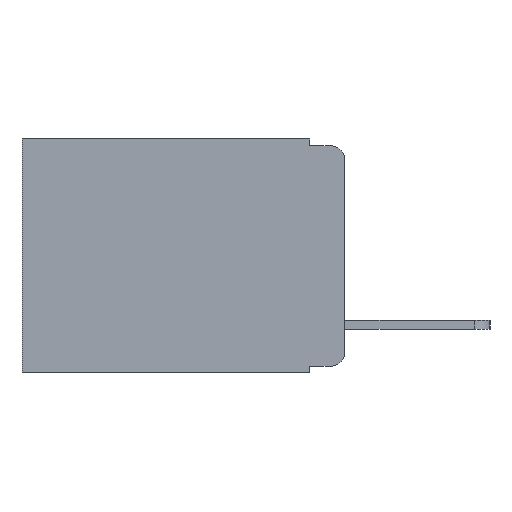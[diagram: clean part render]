
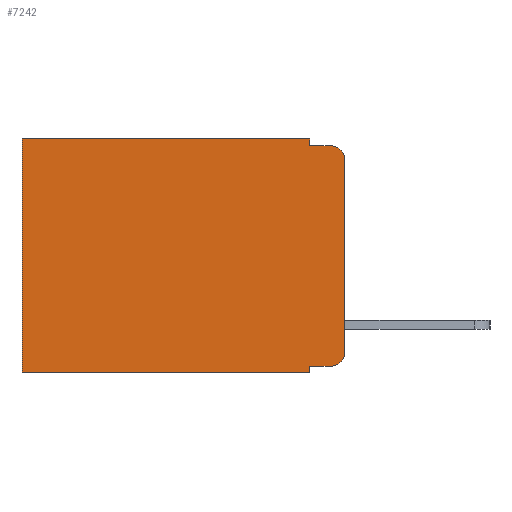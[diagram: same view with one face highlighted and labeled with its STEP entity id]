
A CAD part, left-side view. The second image highlights one B-rep face of the part: STEP entity #7242.
In plain terms, the highlighted planar face has unit normal (-1, 0, 0).
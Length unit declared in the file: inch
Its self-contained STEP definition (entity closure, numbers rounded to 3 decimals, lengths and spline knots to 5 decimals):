
#86 = EDGE_CURVE ( 'NONE', #5661, #2500, #11381, .T. ) ;
#133 = EDGE_LOOP ( 'NONE', ( #2097, #4740, #5464, #5956, #7734, #8742, #486, #1906, #2300, #2674 ) ) ;
#258 = VECTOR ( 'NONE', #10745, 39.37008 ) ;
#445 = VERTEX_POINT ( 'NONE', #5318 ) ;
#486 = ORIENTED_EDGE ( 'NONE', *, *, #9633, .F. ) ;
#683 = LINE ( 'NONE', #10612, #258 ) ;
#869 = VECTOR ( 'NONE', #9114, 39.37008 ) ;
#886 = LINE ( 'NONE', #9125, #869 ) ;
#1081 = DIRECTION ( 'NONE',  ( 0., 0., -1. ) ) ;
#1090 = EDGE_CURVE ( 'NONE', #4045, #10059, #2312, .T. ) ;
#1154 = DIRECTION ( 'NONE',  ( -1., 0., 0. ) ) ;
#1195 = CARTESIAN_POINT ( 'NONE',  ( 0.298, 0.02, -0.03 ) ) ;
#1906 = ORIENTED_EDGE ( 'NONE', *, *, #3934, .F. ) ;
#2074 = VECTOR ( 'NONE', #3559, 39.37008 ) ;
#2097 = ORIENTED_EDGE ( 'NONE', *, *, #8416, .F. ) ;
#2136 = LINE ( 'NONE', #9991, #2074 ) ;
#2219 = AXIS2_PLACEMENT_3D ( 'NONE', #10887, #10707, #10687 ) ;
#2300 = ORIENTED_EDGE ( 'NONE', *, *, #5698, .T. ) ;
#2312 = CIRCLE ( 'NONE', #11860, 0.02 ) ;
#2500 = VERTEX_POINT ( 'NONE', #11569 ) ;
#2591 = EDGE_CURVE ( 'NONE', #4491, #2834, #9206, .T. ) ;
#2674 = ORIENTED_EDGE ( 'NONE', *, *, #1090, .T. ) ;
#2834 = VERTEX_POINT ( 'NONE', #4351 ) ;
#3559 = DIRECTION ( 'NONE',  ( 0., -1., 0. ) ) ;
#3733 = VERTEX_POINT ( 'NONE', #9116 ) ;
#3934 = EDGE_CURVE ( 'NONE', #445, #3733, #886, .T. ) ;
#3970 = CIRCLE ( 'NONE', #11551, 0.02 ) ;
#4045 = VERTEX_POINT ( 'NONE', #9302 ) ;
#4310 = CARTESIAN_POINT ( 'NONE',  ( 0.298, 0., -0.03 ) ) ;
#4351 = CARTESIAN_POINT ( 'NONE',  ( 0.298, 0.473, -0.343 ) ) ;
#4491 = VERTEX_POINT ( 'NONE', #7761 ) ;
#4510 = VERTEX_POINT ( 'NONE', #4310 ) ;
#4536 = EDGE_CURVE ( 'NONE', #7663, #5661, #7298, .T. ) ;
#4740 = ORIENTED_EDGE ( 'NONE', *, *, #9412, .T. ) ;
#4884 = DIRECTION ( 'NONE',  ( 0., -1., 0. ) ) ;
#5318 = CARTESIAN_POINT ( 'NONE',  ( 0.298, 0.051, -0.333 ) ) ;
#5464 = ORIENTED_EDGE ( 'NONE', *, *, #86, .F. ) ;
#5661 = VERTEX_POINT ( 'NONE', #8100 ) ;
#5698 = EDGE_CURVE ( 'NONE', #445, #4045, #2136, .T. ) ;
#5956 = ORIENTED_EDGE ( 'NONE', *, *, #4536, .F. ) ;
#6426 = VECTOR ( 'NONE', #10312, 39.37008 ) ;
#7050 = FACE_OUTER_BOUND ( 'NONE', #133, .T. ) ;
#7242 = ADVANCED_FACE ( 'NONE', ( #7050 ), #10738, .F. ) ;
#7298 = LINE ( 'NONE', #11967, #7513 ) ;
#7364 = CARTESIAN_POINT ( 'NONE',  ( 0.298, 0.473, 0. ) ) ;
#7513 = VECTOR ( 'NONE', #11976, 39.37008 ) ;
#7524 = DIRECTION ( 'NONE',  ( 0., 0., -1. ) ) ;
#7588 = VECTOR ( 'NONE', #11975, 39.37008 ) ;
#7663 = VERTEX_POINT ( 'NONE', #9963 ) ;
#7734 = ORIENTED_EDGE ( 'NONE', *, *, #12021, .T. ) ;
#7761 = CARTESIAN_POINT ( 'NONE',  ( 0.298, 0.473, 0. ) ) ;
#8100 = CARTESIAN_POINT ( 'NONE',  ( 0.298, 0.051, -0.01 ) ) ;
#8416 = EDGE_CURVE ( 'NONE', #4510, #10059, #683, .T. ) ;
#8570 = CARTESIAN_POINT ( 'NONE',  ( 0.298, 0.051, -0.01 ) ) ;
#8742 = ORIENTED_EDGE ( 'NONE', *, *, #2591, .T. ) ;
#9094 = VECTOR ( 'NONE', #7524, 39.37008 ) ;
#9114 = DIRECTION ( 'NONE',  ( 0., 0., -1. ) ) ;
#9116 = CARTESIAN_POINT ( 'NONE',  ( 0.298, 0.051, -0.343 ) ) ;
#9125 = CARTESIAN_POINT ( 'NONE',  ( 0.298, 0.051, 0. ) ) ;
#9206 = LINE ( 'NONE', #7364, #9094 ) ;
#9302 = CARTESIAN_POINT ( 'NONE',  ( 0.298, 0.02, -0.333 ) ) ;
#9412 = EDGE_CURVE ( 'NONE', #4510, #2500, #3970, .T. ) ;
#9633 = EDGE_CURVE ( 'NONE', #3733, #2834, #11682, .T. ) ;
#9963 = CARTESIAN_POINT ( 'NONE',  ( 0.298, 0.051, 0. ) ) ;
#9991 = CARTESIAN_POINT ( 'NONE',  ( 0.298, 0.051, -0.333 ) ) ;
#10059 = VERTEX_POINT ( 'NONE', #10721 ) ;
#10248 = DIRECTION ( 'NONE',  ( -1., 0., 0. ) ) ;
#10291 = CARTESIAN_POINT ( 'NONE',  ( 0.298, 0., 0. ) ) ;
#10312 = DIRECTION ( 'NONE',  ( 0., 1., 0. ) ) ;
#10612 = CARTESIAN_POINT ( 'NONE',  ( 0.298, 0., 0. ) ) ;
#10682 = DIRECTION ( 'NONE',  ( 0., 0., -1. ) ) ;
#10687 = DIRECTION ( 'NONE',  ( 0., 0., -1. ) ) ;
#10707 = DIRECTION ( 'NONE',  ( 1., 0., 0. ) ) ;
#10721 = CARTESIAN_POINT ( 'NONE',  ( 0.298, 0., -0.313 ) ) ;
#10738 = PLANE ( 'NONE',  #2219 ) ;
#10745 = DIRECTION ( 'NONE',  ( 0., 0., -1. ) ) ;
#10887 = CARTESIAN_POINT ( 'NONE',  ( 0.298, 0., 0. ) ) ;
#11017 = VECTOR ( 'NONE', #4884, 39.37008 ) ;
#11296 = CARTESIAN_POINT ( 'NONE',  ( 0.298, 0.02, -0.313 ) ) ;
#11381 = LINE ( 'NONE', #8570, #11017 ) ;
#11551 = AXIS2_PLACEMENT_3D ( 'NONE', #1195, #1154, #1081 ) ;
#11569 = CARTESIAN_POINT ( 'NONE',  ( 0.298, 0.02, -0.01 ) ) ;
#11682 = LINE ( 'NONE', #11814, #7588 ) ;
#11814 = CARTESIAN_POINT ( 'NONE',  ( 0.298, 0., -0.343 ) ) ;
#11860 = AXIS2_PLACEMENT_3D ( 'NONE', #11296, #10248, #10682 ) ;
#11942 = LINE ( 'NONE', #10291, #6426 ) ;
#11967 = CARTESIAN_POINT ( 'NONE',  ( 0.298, 0.051, 0. ) ) ;
#11975 = DIRECTION ( 'NONE',  ( 0., 1., 0. ) ) ;
#11976 = DIRECTION ( 'NONE',  ( 0., 0., -1. ) ) ;
#12021 = EDGE_CURVE ( 'NONE', #7663, #4491, #11942, .T. ) ;
